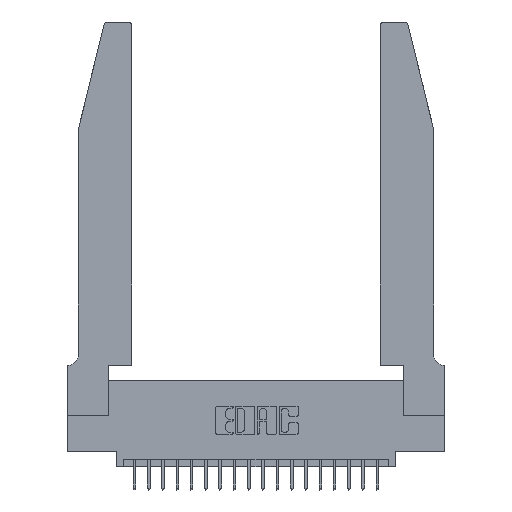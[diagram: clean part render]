
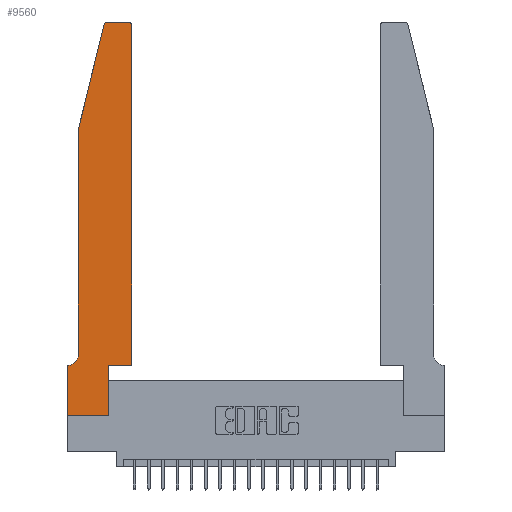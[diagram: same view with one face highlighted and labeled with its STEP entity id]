
A CAD part, top view. The second image highlights one B-rep face of the part: STEP entity #9560.
In plain terms, the highlighted planar face has unit normal (0, 0, 1).
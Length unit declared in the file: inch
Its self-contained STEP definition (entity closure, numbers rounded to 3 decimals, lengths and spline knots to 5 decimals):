
#44 = AXIS2_PLACEMENT_3D ( 'NONE', #18443, #8148, #20160 ) ;
#190 = VERTEX_POINT ( 'NONE', #1522 ) ;
#274 = DIRECTION ( 'NONE',  ( 0., -1., 0. ) ) ;
#294 = DIRECTION ( 'NONE',  ( 0., 0., -1. ) ) ;
#308 = CARTESIAN_POINT ( 'NONE',  ( 0., 0., 0.37 ) ) ;
#408 = EDGE_CURVE ( 'NONE', #11556, #19247, #3352, .T. ) ;
#759 = EDGE_CURVE ( 'NONE', #19247, #13878, #8291, .T. ) ;
#1031 = EDGE_CURVE ( 'NONE', #4955, #190, #11525, .T. ) ;
#1522 = CARTESIAN_POINT ( 'NONE',  ( 0.0755, 2., 0.37 ) ) ;
#1932 = DIRECTION ( 'NONE',  ( 0., -1., 0. ) ) ;
#1982 = ORIENTED_EDGE ( 'NONE', *, *, #2530, .T. ) ;
#2370 = VECTOR ( 'NONE', #3719, 39.37008 ) ;
#2392 = CARTESIAN_POINT ( 'NONE',  ( 0.2605, 2.75, 0.37 ) ) ;
#2530 = EDGE_CURVE ( 'NONE', #13878, #22140, #12553, .T. ) ;
#2815 = CIRCLE ( 'NONE', #14218, 0.03 ) ;
#2881 = ORIENTED_EDGE ( 'NONE', *, *, #1031, .T. ) ;
#3116 = VECTOR ( 'NONE', #19502, 39.37008 ) ;
#3157 = EDGE_CURVE ( 'NONE', #18691, #14397, #9805, .T. ) ;
#3313 = EDGE_CURVE ( 'NONE', #14397, #15803, #7130, .T. ) ;
#3352 = LINE ( 'NONE', #19634, #7358 ) ;
#3561 = EDGE_CURVE ( 'NONE', #15803, #4955, #2815, .T. ) ;
#3681 = CARTESIAN_POINT ( 'NONE',  ( 0.4505, 0.35, 0.37 ) ) ;
#3719 = DIRECTION ( 'NONE',  ( -0.239, -0.971, 0. ) ) ;
#3858 = LINE ( 'NONE', #3681, #16435 ) ;
#3870 = DIRECTION ( 'NONE',  ( -1., 0., 0. ) ) ;
#4589 = CARTESIAN_POINT ( 'NONE',  ( 0.2865, 0., 0.37 ) ) ;
#4675 = CARTESIAN_POINT ( 'NONE',  ( 0.4205, 2.75, 0.37 ) ) ;
#4677 = VECTOR ( 'NONE', #1932, 39.37008 ) ;
#4866 = ORIENTED_EDGE ( 'NONE', *, *, #11557, .T. ) ;
#4955 = VERTEX_POINT ( 'NONE', #8410 ) ;
#5123 = EDGE_CURVE ( 'NONE', #190, #11767, #9180, .T. ) ;
#5301 = VECTOR ( 'NONE', #20897, 39.37008 ) ;
#5528 = CARTESIAN_POINT ( 'NONE',  ( 0.4205, 2.72, 0.37 ) ) ;
#5695 = ORIENTED_EDGE ( 'NONE', *, *, #9869, .T. ) ;
#6033 = CARTESIAN_POINT ( 'NONE',  ( 0.0755, 2., 0.37 ) ) ;
#6261 = ORIENTED_EDGE ( 'NONE', *, *, #3561, .T. ) ;
#6660 = VECTOR ( 'NONE', #14290, 39.37008 ) ;
#7130 = LINE ( 'NONE', #2392, #3116 ) ;
#7224 = DIRECTION ( 'NONE',  ( 1., 0., 0. ) ) ;
#7358 = VECTOR ( 'NONE', #3870, 39.37008 ) ;
#7521 = CARTESIAN_POINT ( 'NONE',  ( 0.0755, 0.42, 0.37 ) ) ;
#7631 = CIRCLE ( 'NONE', #19735, 0.07 ) ;
#8148 = DIRECTION ( 'NONE',  ( 0., 0., 1. ) ) ;
#8291 = LINE ( 'NONE', #308, #16365 ) ;
#8410 = CARTESIAN_POINT ( 'NONE',  ( 0.25487, 2.72718, 0.37 ) ) ;
#8661 = ORIENTED_EDGE ( 'NONE', *, *, #9316, .T. ) ;
#9180 = LINE ( 'NONE', #12190, #4677 ) ;
#9276 = LINE ( 'NONE', #14058, #5301 ) ;
#9316 = EDGE_CURVE ( 'NONE', #11604, #16698, #9276, .T. ) ;
#9560 = ADVANCED_FACE ( 'NONE', ( #17597 ), #15009, .T. ) ;
#9805 = CIRCLE ( 'NONE', #13501, 0.03 ) ;
#9869 = EDGE_CURVE ( 'NONE', #11767, #11556, #7631, .T. ) ;
#9894 = DIRECTION ( 'NONE',  ( 0., 0., 1. ) ) ;
#10137 = CARTESIAN_POINT ( 'NONE',  ( 0.4505, 0.35, 0.37 ) ) ;
#10434 = ORIENTED_EDGE ( 'NONE', *, *, #759, .T. ) ;
#10599 = CARTESIAN_POINT ( 'NONE',  ( 0.2865, 0.35, 0.37 ) ) ;
#10603 = CARTESIAN_POINT ( 'NONE',  ( 0., 0., 0.37 ) ) ;
#10688 = CARTESIAN_POINT ( 'NONE',  ( 0.0055, 0.42, 0.37 ) ) ;
#11204 = CARTESIAN_POINT ( 'NONE',  ( 0., 0.35, 0.37 ) ) ;
#11525 = LINE ( 'NONE', #6033, #2370 ) ;
#11556 = VERTEX_POINT ( 'NONE', #15648 ) ;
#11557 = EDGE_CURVE ( 'NONE', #16698, #18691, #3858, .T. ) ;
#11604 = VERTEX_POINT ( 'NONE', #10599 ) ;
#11767 = VERTEX_POINT ( 'NONE', #7521 ) ;
#11783 = LINE ( 'NONE', #19423, #6660 ) ;
#11994 = DIRECTION ( 'NONE',  ( 1., 0., 0. ) ) ;
#12190 = CARTESIAN_POINT ( 'NONE',  ( 0.0755, 2., 0.37 ) ) ;
#12460 = DIRECTION ( 'NONE',  ( -1., 0., 0. ) ) ;
#12553 = LINE ( 'NONE', #10603, #16016 ) ;
#12648 = ORIENTED_EDGE ( 'NONE', *, *, #3157, .T. ) ;
#13501 = AXIS2_PLACEMENT_3D ( 'NONE', #5528, #17497, #7224 ) ;
#13878 = VERTEX_POINT ( 'NONE', #18610 ) ;
#14058 = CARTESIAN_POINT ( 'NONE',  ( 0.4505, 0.35, 0.37 ) ) ;
#14218 = AXIS2_PLACEMENT_3D ( 'NONE', #20172, #9894, #21867 ) ;
#14290 = DIRECTION ( 'NONE',  ( 0., 1., 0. ) ) ;
#14397 = VERTEX_POINT ( 'NONE', #4675 ) ;
#14668 = ORIENTED_EDGE ( 'NONE', *, *, #5123, .T. ) ;
#15009 = PLANE ( 'NONE',  #44 ) ;
#15648 = CARTESIAN_POINT ( 'NONE',  ( 0.0055, 0.35, 0.37 ) ) ;
#15803 = VERTEX_POINT ( 'NONE', #16873 ) ;
#16016 = VECTOR ( 'NONE', #11994, 39.37008 ) ;
#16365 = VECTOR ( 'NONE', #274, 39.37008 ) ;
#16435 = VECTOR ( 'NONE', #17381, 39.37008 ) ;
#16698 = VERTEX_POINT ( 'NONE', #10137 ) ;
#16873 = CARTESIAN_POINT ( 'NONE',  ( 0.284, 2.75, 0.37 ) ) ;
#16912 = EDGE_CURVE ( 'NONE', #22140, #11604, #11783, .T. ) ;
#17123 = CARTESIAN_POINT ( 'NONE',  ( 0.4505, 2.72, 0.37 ) ) ;
#17381 = DIRECTION ( 'NONE',  ( 0., 1., 0. ) ) ;
#17497 = DIRECTION ( 'NONE',  ( 0., 0., 1. ) ) ;
#17597 = FACE_OUTER_BOUND ( 'NONE', #19604, .T. ) ;
#18443 = CARTESIAN_POINT ( 'NONE',  ( 0., 0.35, 0.37 ) ) ;
#18610 = CARTESIAN_POINT ( 'NONE',  ( 0., 0., 0.37 ) ) ;
#18691 = VERTEX_POINT ( 'NONE', #17123 ) ;
#19247 = VERTEX_POINT ( 'NONE', #11204 ) ;
#19423 = CARTESIAN_POINT ( 'NONE',  ( 0.2865, 0.35, 0.37 ) ) ;
#19502 = DIRECTION ( 'NONE',  ( -1., 0., 0. ) ) ;
#19507 = ORIENTED_EDGE ( 'NONE', *, *, #16912, .T. ) ;
#19604 = EDGE_LOOP ( 'NONE', ( #22290, #6261, #2881, #14668, #5695, #20147, #10434, #1982, #19507, #8661, #4866, #12648 ) ) ;
#19634 = CARTESIAN_POINT ( 'NONE',  ( 0.0755, 0.35, 0.37 ) ) ;
#19735 = AXIS2_PLACEMENT_3D ( 'NONE', #10688, #294, #12460 ) ;
#20147 = ORIENTED_EDGE ( 'NONE', *, *, #408, .T. ) ;
#20160 = DIRECTION ( 'NONE',  ( 1., 0., 0. ) ) ;
#20172 = CARTESIAN_POINT ( 'NONE',  ( 0.284, 2.72, 0.37 ) ) ;
#20897 = DIRECTION ( 'NONE',  ( 1., 0., 0. ) ) ;
#21867 = DIRECTION ( 'NONE',  ( 1., 0., 0. ) ) ;
#22140 = VERTEX_POINT ( 'NONE', #4589 ) ;
#22290 = ORIENTED_EDGE ( 'NONE', *, *, #3313, .T. ) ;
